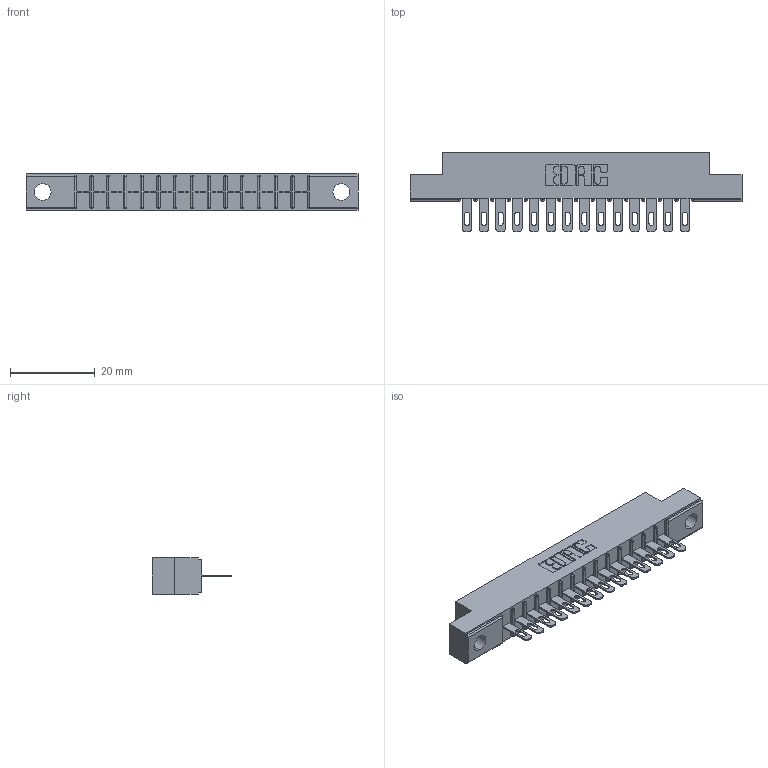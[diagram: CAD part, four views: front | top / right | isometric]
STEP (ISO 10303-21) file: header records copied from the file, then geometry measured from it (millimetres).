
FILE_DESCRIPTION (( 'STEP AP203' ), '1' );
FILE_NAME ('356-014-500-104.STEP', '2018-08-01T19:02:43', ( '' ), ( '' ), 'SwSTEP 2.0', 'SolidWorks 2016', '' );
FILE_SCHEMA (( 'CONFIG_CONTROL_DESIGN' ));
Length unit declared in the file: inch
Products named in the file (3): 306 Part_.156 Dia; 306-290-001_100; 356-014-500-104
Assembly tree (15 placements, depth 2):
  356-014-500-104
    306 Part_.156 Dia
    306-290-001_100  x14
Bounding box: 78.49 x 18.87 x 8.71 mm (x, y, z)
Volume: 5267.6 mm3; surface area: 7631.2 mm2
Topology: 15 solids, 15 shells, 1194 faces, 3362 edges, 2164 vertices
Faces by surface type: plane 782, cylinder 356, sphere 56
Entity records: 17265 total; most frequent: CARTESIAN_POINT 2899, ORIENTED_EDGE 2868, DIRECTION 2854, EDGE_CURVE 1434, VECTOR 1112, LINE 1112, VERTEX_POINT 916, AXIS2_PLACEMENT_3D 871
